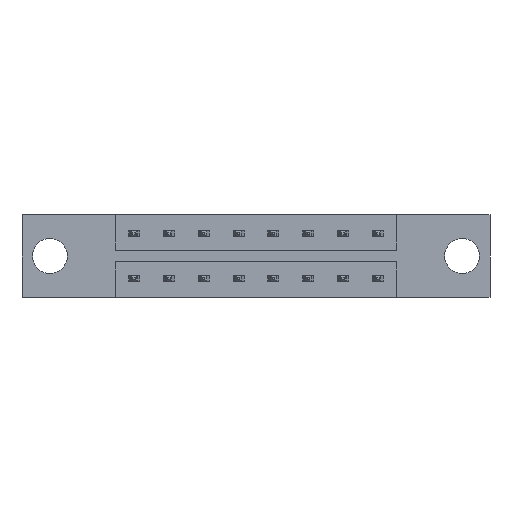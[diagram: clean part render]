
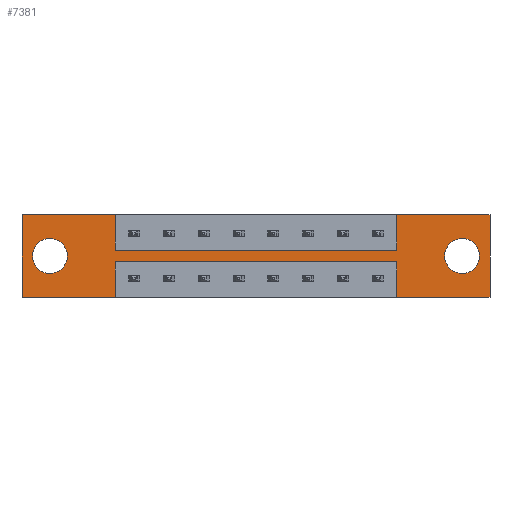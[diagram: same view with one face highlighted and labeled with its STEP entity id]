
A CAD part, front view. The second image highlights one B-rep face of the part: STEP entity #7381.
In plain terms, the highlighted planar face has unit normal (0, -1, 0).
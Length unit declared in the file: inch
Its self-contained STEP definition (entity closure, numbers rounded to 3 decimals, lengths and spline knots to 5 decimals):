
#104 = VERTEX_POINT ( 'NONE', #2695 ) ;
#149 = EDGE_LOOP ( 'NONE', ( #8820, #7134 ) ) ;
#183 = VECTOR ( 'NONE', #970, 39.37008 ) ;
#318 = VERTEX_POINT ( 'NONE', #4298 ) ;
#341 = CARTESIAN_POINT ( 'NONE',  ( 0., 0., -0.37 ) ) ;
#498 = VERTEX_POINT ( 'NONE', #8624 ) ;
#502 = CARTESIAN_POINT ( 'NONE',  ( 0.4175, 0., -0.1585 ) ) ;
#542 = CARTESIAN_POINT ( 'NONE',  ( 0.125, 0., -0.185 ) ) ;
#753 = CARTESIAN_POINT ( 'NONE',  ( 2.096, 0., 0. ) ) ;
#769 = DIRECTION ( 'NONE',  ( 0., 0., 1. ) ) ;
#823 = EDGE_CURVE ( 'NONE', #9512, #104, #8804, .T. ) ;
#901 = FACE_BOUND ( 'NONE', #149, .T. ) ;
#928 = DIRECTION ( 'NONE',  ( 0., 0., -1. ) ) ;
#948 = EDGE_CURVE ( 'NONE', #8203, #9388, #4015, .T. ) ;
#970 = DIRECTION ( 'NONE',  ( 1., 0., 0. ) ) ;
#1068 = CARTESIAN_POINT ( 'NONE',  ( 0.125, 0., -0.107 ) ) ;
#1081 = DIRECTION ( 'NONE',  ( 0., 1., 0. ) ) ;
#1088 = AXIS2_PLACEMENT_3D ( 'NONE', #6466, #1081, #928 ) ;
#1191 = EDGE_CURVE ( 'NONE', #3446, #7967, #6329, .T. ) ;
#1204 = DIRECTION ( 'NONE',  ( -1., 0., 0. ) ) ;
#1221 = EDGE_CURVE ( 'NONE', #7135, #498, #3667, .T. ) ;
#1277 = CARTESIAN_POINT ( 'NONE',  ( 0., 0., -0.37 ) ) ;
#1399 = LINE ( 'NONE', #9257, #5149 ) ;
#1410 = VECTOR ( 'NONE', #2753, 39.37008 ) ;
#1417 = VECTOR ( 'NONE', #4579, 39.37008 ) ;
#1476 = AXIS2_PLACEMENT_3D ( 'NONE', #7173, #8651, #4290 ) ;
#1586 = LINE ( 'NONE', #3969, #5308 ) ;
#1679 = ORIENTED_EDGE ( 'NONE', *, *, #1736, .T. ) ;
#1736 = EDGE_CURVE ( 'NONE', #9194, #7974, #5367, .T. ) ;
#1774 = VECTOR ( 'NONE', #5383, 39.37008 ) ;
#1884 = VECTOR ( 'NONE', #3776, 39.37008 ) ;
#1969 = VECTOR ( 'NONE', #3597, 39.37008 ) ;
#2004 = CARTESIAN_POINT ( 'NONE',  ( 0.4175, 0., -0.2115 ) ) ;
#2050 = DIRECTION ( 'NONE',  ( -1., 0., 0. ) ) ;
#2095 = AXIS2_PLACEMENT_3D ( 'NONE', #7261, #2836, #7991 ) ;
#2144 = ORIENTED_EDGE ( 'NONE', *, *, #7315, .F. ) ;
#2152 = ORIENTED_EDGE ( 'NONE', *, *, #6859, .F. ) ;
#2273 = LINE ( 'NONE', #1277, #6025 ) ;
#2306 = CARTESIAN_POINT ( 'NONE',  ( 1.6785, 0., -0.1585 ) ) ;
#2512 = ORIENTED_EDGE ( 'NONE', *, *, #823, .F. ) ;
#2544 = CIRCLE ( 'NONE', #6585, 0.078 ) ;
#2695 = CARTESIAN_POINT ( 'NONE',  ( 0.4175, 0., -0.2115 ) ) ;
#2701 = ORIENTED_EDGE ( 'NONE', *, *, #7865, .F. ) ;
#2703 = FACE_OUTER_BOUND ( 'NONE', #4079, .T. ) ;
#2753 = DIRECTION ( 'NONE',  ( 0., 0., -1. ) ) ;
#2793 = EDGE_CURVE ( 'NONE', #8520, #7284, #9540, .T. ) ;
#2836 = DIRECTION ( 'NONE',  ( 0., 1., 0. ) ) ;
#2861 = LINE ( 'NONE', #4550, #6579 ) ;
#2890 = VECTOR ( 'NONE', #9453, 39.37008 ) ;
#3137 = EDGE_CURVE ( 'NONE', #7974, #9194, #2544, .T. ) ;
#3446 = VERTEX_POINT ( 'NONE', #2306 ) ;
#3597 = DIRECTION ( 'NONE',  ( 0., 0., -1. ) ) ;
#3667 = CIRCLE ( 'NONE', #1088, 0.078 ) ;
#3747 = EDGE_LOOP ( 'NONE', ( #6807, #1679 ) ) ;
#3776 = DIRECTION ( 'NONE',  ( 0., 0., 1. ) ) ;
#3862 = CARTESIAN_POINT ( 'NONE',  ( 0.4175, 0., -0.37 ) ) ;
#3872 = CARTESIAN_POINT ( 'NONE',  ( 1.6785, 0., -0.1585 ) ) ;
#3932 = DIRECTION ( 'NONE',  ( 0., 0., 1. ) ) ;
#3969 = CARTESIAN_POINT ( 'NONE',  ( 1.6785, 0., -0.2115 ) ) ;
#4015 = LINE ( 'NONE', #502, #1774 ) ;
#4040 = ORIENTED_EDGE ( 'NONE', *, *, #948, .F. ) ;
#4079 = EDGE_LOOP ( 'NONE', ( #7599, #5900, #6352, #2144, #4687, #2701, #4040, #7252, #6244, #5653, #2152, #2512 ) ) ;
#4104 = CARTESIAN_POINT ( 'NONE',  ( 1.6785, 0., 0. ) ) ;
#4184 = EDGE_CURVE ( 'NONE', #318, #9512, #1586, .T. ) ;
#4219 = VERTEX_POINT ( 'NONE', #3862 ) ;
#4290 = DIRECTION ( 'NONE',  ( 0., 0., -1. ) ) ;
#4298 = CARTESIAN_POINT ( 'NONE',  ( 1.6785, 0., -0.37 ) ) ;
#4502 = CIRCLE ( 'NONE', #2095, 0.078 ) ;
#4550 = CARTESIAN_POINT ( 'NONE',  ( 0., 0., 0. ) ) ;
#4570 = EDGE_CURVE ( 'NONE', #7284, #318, #2273, .T. ) ;
#4579 = DIRECTION ( 'NONE',  ( -1., 0., 0. ) ) ;
#4635 = CARTESIAN_POINT ( 'NONE',  ( 1.6785, 0., -0.2115 ) ) ;
#4687 = ORIENTED_EDGE ( 'NONE', *, *, #1191, .F. ) ;
#4698 = FACE_BOUND ( 'NONE', #3747, .T. ) ;
#4929 = LINE ( 'NONE', #7971, #6898 ) ;
#4996 = EDGE_CURVE ( 'NONE', #6982, #8203, #6471, .T. ) ;
#5149 = VECTOR ( 'NONE', #6419, 39.37008 ) ;
#5153 = EDGE_CURVE ( 'NONE', #8015, #6982, #2861, .T. ) ;
#5308 = VECTOR ( 'NONE', #3932, 39.37008 ) ;
#5367 = CIRCLE ( 'NONE', #5967, 0.078 ) ;
#5383 = DIRECTION ( 'NONE',  ( 0., 0., -1. ) ) ;
#5470 = CARTESIAN_POINT ( 'NONE',  ( 0.4175, 0., -0.1585 ) ) ;
#5600 = EDGE_CURVE ( 'NONE', #498, #7135, #4502, .T. ) ;
#5653 = ORIENTED_EDGE ( 'NONE', *, *, #6910, .F. ) ;
#5842 = DIRECTION ( 'NONE',  ( 0., 0., 1. ) ) ;
#5900 = ORIENTED_EDGE ( 'NONE', *, *, #4570, .F. ) ;
#5967 = AXIS2_PLACEMENT_3D ( 'NONE', #542, #9464, #8248 ) ;
#6025 = VECTOR ( 'NONE', #1204, 39.37008 ) ;
#6202 = CARTESIAN_POINT ( 'NONE',  ( 1.971, 0., -0.263 ) ) ;
#6244 = ORIENTED_EDGE ( 'NONE', *, *, #5153, .F. ) ;
#6329 = LINE ( 'NONE', #3872, #1884 ) ;
#6352 = ORIENTED_EDGE ( 'NONE', *, *, #2793, .F. ) ;
#6389 = CARTESIAN_POINT ( 'NONE',  ( 2.096, 0., -0.37 ) ) ;
#6419 = DIRECTION ( 'NONE',  ( 1., 0., 0. ) ) ;
#6459 = CARTESIAN_POINT ( 'NONE',  ( 0.4175, 0., -0.2115 ) ) ;
#6466 = CARTESIAN_POINT ( 'NONE',  ( 1.971, 0., -0.185 ) ) ;
#6471 = LINE ( 'NONE', #8003, #2890 ) ;
#6579 = VECTOR ( 'NONE', #769, 39.37008 ) ;
#6585 = AXIS2_PLACEMENT_3D ( 'NONE', #9152, #9208, #5842 ) ;
#6591 = CARTESIAN_POINT ( 'NONE',  ( 0.4175, 0., 0. ) ) ;
#6807 = ORIENTED_EDGE ( 'NONE', *, *, #3137, .T. ) ;
#6859 = EDGE_CURVE ( 'NONE', #104, #4219, #7349, .T. ) ;
#6898 = VECTOR ( 'NONE', #2050, 39.37008 ) ;
#6910 = EDGE_CURVE ( 'NONE', #4219, #8015, #4929, .T. ) ;
#6982 = VERTEX_POINT ( 'NONE', #8903 ) ;
#7134 = ORIENTED_EDGE ( 'NONE', *, *, #1221, .T. ) ;
#7135 = VERTEX_POINT ( 'NONE', #6202 ) ;
#7173 = CARTESIAN_POINT ( 'NONE',  ( 0., 0., -0.37 ) ) ;
#7252 = ORIENTED_EDGE ( 'NONE', *, *, #4996, .F. ) ;
#7261 = CARTESIAN_POINT ( 'NONE',  ( 1.971, 0., -0.185 ) ) ;
#7284 = VERTEX_POINT ( 'NONE', #6389 ) ;
#7315 = EDGE_CURVE ( 'NONE', #7967, #8520, #1399, .T. ) ;
#7349 = LINE ( 'NONE', #6459, #1410 ) ;
#7381 = ADVANCED_FACE ( 'NONE', ( #901, #4698, #2703 ), #7929, .T. ) ;
#7599 = ORIENTED_EDGE ( 'NONE', *, *, #4184, .F. ) ;
#7691 = CARTESIAN_POINT ( 'NONE',  ( 2.096, 0., 0. ) ) ;
#7865 = EDGE_CURVE ( 'NONE', #9388, #3446, #7891, .T. ) ;
#7891 = LINE ( 'NONE', #5470, #183 ) ;
#7929 = PLANE ( 'NONE',  #1476 ) ;
#7967 = VERTEX_POINT ( 'NONE', #4104 ) ;
#7971 = CARTESIAN_POINT ( 'NONE',  ( 0., 0., -0.37 ) ) ;
#7974 = VERTEX_POINT ( 'NONE', #1068 ) ;
#7991 = DIRECTION ( 'NONE',  ( 0., 0., -1. ) ) ;
#8003 = CARTESIAN_POINT ( 'NONE',  ( 0., 0., 0. ) ) ;
#8015 = VERTEX_POINT ( 'NONE', #341 ) ;
#8203 = VERTEX_POINT ( 'NONE', #6591 ) ;
#8248 = DIRECTION ( 'NONE',  ( 0., 0., 1. ) ) ;
#8520 = VERTEX_POINT ( 'NONE', #7691 ) ;
#8624 = CARTESIAN_POINT ( 'NONE',  ( 1.971, 0., -0.107 ) ) ;
#8651 = DIRECTION ( 'NONE',  ( 0., -1., 0. ) ) ;
#8804 = LINE ( 'NONE', #2004, #1417 ) ;
#8820 = ORIENTED_EDGE ( 'NONE', *, *, #5600, .T. ) ;
#8903 = CARTESIAN_POINT ( 'NONE',  ( 0., 0., 0. ) ) ;
#9152 = CARTESIAN_POINT ( 'NONE',  ( 0.125, 0., -0.185 ) ) ;
#9194 = VERTEX_POINT ( 'NONE', #9339 ) ;
#9208 = DIRECTION ( 'NONE',  ( 0., 1., 0. ) ) ;
#9257 = CARTESIAN_POINT ( 'NONE',  ( 0., 0., 0. ) ) ;
#9339 = CARTESIAN_POINT ( 'NONE',  ( 0.125, 0., -0.263 ) ) ;
#9388 = VERTEX_POINT ( 'NONE', #9536 ) ;
#9453 = DIRECTION ( 'NONE',  ( 1., 0., 0. ) ) ;
#9464 = DIRECTION ( 'NONE',  ( 0., 1., 0. ) ) ;
#9512 = VERTEX_POINT ( 'NONE', #4635 ) ;
#9536 = CARTESIAN_POINT ( 'NONE',  ( 0.4175, 0., -0.1585 ) ) ;
#9540 = LINE ( 'NONE', #753, #1969 ) ;
